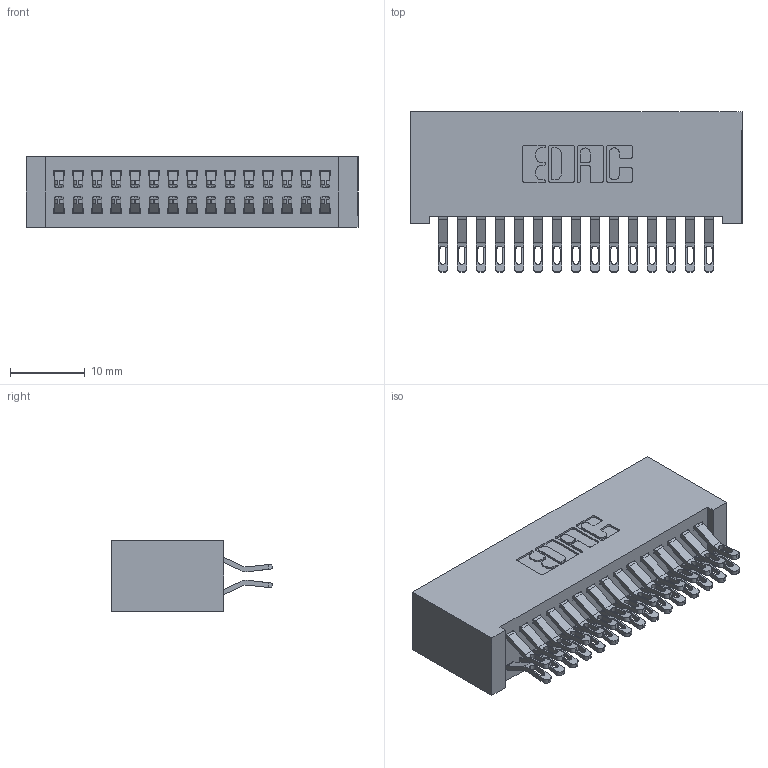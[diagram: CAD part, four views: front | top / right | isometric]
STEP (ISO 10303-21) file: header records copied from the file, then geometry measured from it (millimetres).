
FILE_DESCRIPTION (( 'STEP AP203' ), '1' );
FILE_NAME ('342-030-555-201.STEP', '2018-08-11T15:45:16', ( '' ), ( '' ), 'SwSTEP 2.0', 'SolidWorks 2016', '' );
FILE_SCHEMA (( 'CONFIG_CONTROL_DESIGN' ));
Length unit declared in the file: inch
Products named in the file (3): 342 Part_Lugless; 345-292-001_555 Tail; 342-030-555-201
Assembly tree (31 placements, depth 2):
  342-030-555-201
    342 Part_Lugless
    345-292-001_555 Tail  x30
Bounding box: 44.35 x 21.47 x 9.4 mm (x, y, z)
Volume: 4379.8 mm3; surface area: 7200.4 mm2
Topology: 31 solids, 31 shells, 1842 faces, 5765 edges, 3842 vertices
Faces by surface type: plane 1082, cylinder 760
Entity records: 13059 total; most frequent: CARTESIAN_POINT 2228, ORIENTED_EDGE 2134, DIRECTION 1915, EDGE_CURVE 1067, VECTOR 927, LINE 927, VERTEX_POINT 710, AXIS2_PLACEMENT_3D 494
